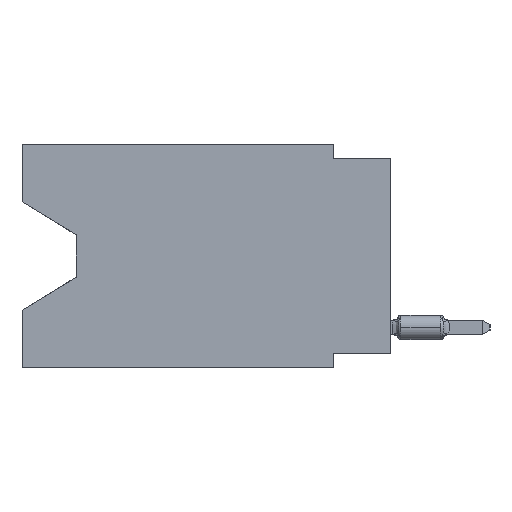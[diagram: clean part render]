
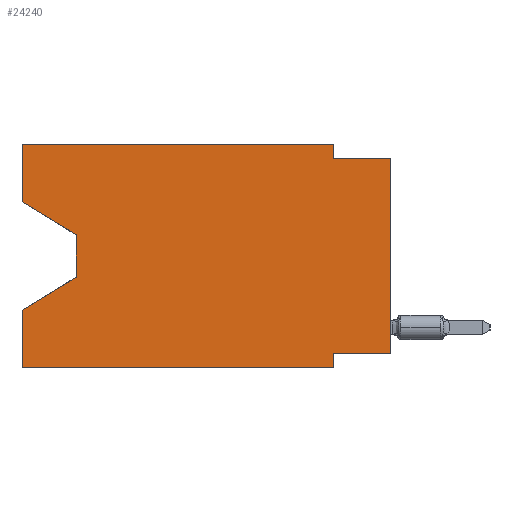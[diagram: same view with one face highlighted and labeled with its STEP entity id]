
A CAD part, left-side view. The second image highlights one B-rep face of the part: STEP entity #24240.
In plain terms, the highlighted planar face has unit normal (-1, 0, 0).
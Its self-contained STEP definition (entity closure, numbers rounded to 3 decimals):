
#132 = ORIENTED_EDGE ( 'NONE', *, *, #22557, .F. ) ;
#424 = EDGE_CURVE ( 'NONE', #26440, #10330, #9604, .T. ) ;
#500 = EDGE_CURVE ( 'NONE', #512, #4756, #3976, .T. ) ;
#512 = VERTEX_POINT ( 'NONE', #6224 ) ;
#558 = ORIENTED_EDGE ( 'NONE', *, *, #12560, .F. ) ;
#1077 = VERTEX_POINT ( 'NONE', #13866 ) ;
#1484 = EDGE_CURVE ( 'NONE', #2881, #12693, #14438, .T. ) ;
#2735 = CARTESIAN_POINT ( 'NONE',  ( 0., 13.97, -5.893 ) ) ;
#2881 = VERTEX_POINT ( 'NONE', #2735 ) ;
#3331 = ORIENTED_EDGE ( 'NONE', *, *, #6222, .F. ) ;
#3629 = VECTOR ( 'NONE', #13772, 1000. ) ;
#3734 = CARTESIAN_POINT ( 'NONE',  ( 0., 16.383, 0. ) ) ;
#3819 = ORIENTED_EDGE ( 'NONE', *, *, #23632, .F. ) ;
#3976 = LINE ( 'NONE', #12163, #6084 ) ;
#4308 = EDGE_CURVE ( 'NONE', #27775, #18327, #11653, .T. ) ;
#4413 = DIRECTION ( 'NONE',  ( 0., 0., -1. ) ) ;
#4453 = DIRECTION ( 'NONE',  ( 0., -1., 0. ) ) ;
#4756 = VERTEX_POINT ( 'NONE', #18749 ) ;
#4885 = CARTESIAN_POINT ( 'NONE',  ( 0., 16.383, 0. ) ) ;
#5933 = DIRECTION ( 'NONE',  ( 0., 0., -1. ) ) ;
#6084 = VECTOR ( 'NONE', #5933, 1000. ) ;
#6222 = EDGE_CURVE ( 'NONE', #9486, #10330, #21521, .T. ) ;
#6224 = CARTESIAN_POINT ( 'NONE',  ( 0., 2.54, -9.271 ) ) ;
#7427 = ORIENTED_EDGE ( 'NONE', *, *, #14307, .T. ) ;
#7563 = CARTESIAN_POINT ( 'NONE',  ( 0., 0., -9.271 ) ) ;
#8076 = CARTESIAN_POINT ( 'NONE',  ( 0., 2.54, 0. ) ) ;
#8082 = ORIENTED_EDGE ( 'NONE', *, *, #424, .T. ) ;
#8189 = LINE ( 'NONE', #16778, #14380 ) ;
#8214 = CARTESIAN_POINT ( 'NONE',  ( 0., 13.97, -5.893 ) ) ;
#8328 = EDGE_CURVE ( 'NONE', #18327, #9486, #8189, .T. ) ;
#9486 = VERTEX_POINT ( 'NONE', #22863 ) ;
#9604 = LINE ( 'NONE', #26800, #26778 ) ;
#9641 = VECTOR ( 'NONE', #24314, 1000. ) ;
#9661 = ORIENTED_EDGE ( 'NONE', *, *, #20714, .T. ) ;
#9950 = CARTESIAN_POINT ( 'NONE',  ( 0., 16.383, 0. ) ) ;
#10283 = CARTESIAN_POINT ( 'NONE',  ( 0., 16.383, -9.906 ) ) ;
#10330 = VERTEX_POINT ( 'NONE', #20951 ) ;
#10488 = LINE ( 'NONE', #23344, #19471 ) ;
#10808 = LINE ( 'NONE', #12367, #14360 ) ;
#11653 = LINE ( 'NONE', #4885, #9641 ) ;
#12163 = CARTESIAN_POINT ( 'NONE',  ( 0., 2.54, -9.906 ) ) ;
#12346 = VECTOR ( 'NONE', #23282, 1000. ) ;
#12367 = CARTESIAN_POINT ( 'NONE',  ( 0., 0., -9.271 ) ) ;
#12443 = VERTEX_POINT ( 'NONE', #27869 ) ;
#12560 = EDGE_CURVE ( 'NONE', #26440, #512, #10808, .T. ) ;
#12693 = VERTEX_POINT ( 'NONE', #24323 ) ;
#13282 = FACE_OUTER_BOUND ( 'NONE', #19927, .T. ) ;
#13679 = ORIENTED_EDGE ( 'NONE', *, *, #20221, .T. ) ;
#13772 = DIRECTION ( 'NONE',  ( 0., 0., 1. ) ) ;
#13803 = VECTOR ( 'NONE', #14160, 1000. ) ;
#13866 = CARTESIAN_POINT ( 'NONE',  ( 0., 16.383, -2.546 ) ) ;
#14160 = DIRECTION ( 'NONE',  ( 0., 0.855, -0.519 ) ) ;
#14307 = EDGE_CURVE ( 'NONE', #12443, #4756, #15225, .T. ) ;
#14360 = VECTOR ( 'NONE', #25306, 1000. ) ;
#14380 = VECTOR ( 'NONE', #24951, 1000. ) ;
#14438 = LINE ( 'NONE', #8214, #13803 ) ;
#15225 = LINE ( 'NONE', #10283, #21953 ) ;
#16382 = VERTEX_POINT ( 'NONE', #19220 ) ;
#16387 = DIRECTION ( 'NONE',  ( 0., 0., 1. ) ) ;
#16778 = CARTESIAN_POINT ( 'NONE',  ( 0., 2.54, 0. ) ) ;
#17148 = CARTESIAN_POINT ( 'NONE',  ( 0., 13.97, -4.013 ) ) ;
#17267 = CARTESIAN_POINT ( 'NONE',  ( 0., 0., -0.635 ) ) ;
#18327 = VERTEX_POINT ( 'NONE', #8076 ) ;
#18339 = AXIS2_PLACEMENT_3D ( 'NONE', #21888, #26368, #4413 ) ;
#18749 = CARTESIAN_POINT ( 'NONE',  ( 0., 2.54, -9.906 ) ) ;
#18832 = DIRECTION ( 'NONE',  ( 0., 0., 1. ) ) ;
#18903 = CARTESIAN_POINT ( 'NONE',  ( 0., 16.383, -2.546 ) ) ;
#19220 = CARTESIAN_POINT ( 'NONE',  ( 0., 13.97, -4.013 ) ) ;
#19272 = DIRECTION ( 'NONE',  ( 0., 0., -1. ) ) ;
#19451 = ORIENTED_EDGE ( 'NONE', *, *, #500, .F. ) ;
#19471 = VECTOR ( 'NONE', #18832, 1000. ) ;
#19927 = EDGE_LOOP ( 'NONE', ( #13679, #9661, #20577, #132, #7427, #19451, #558, #8082, #3331, #20949, #26151, #3819 ) ) ;
#20221 = EDGE_CURVE ( 'NONE', #1077, #16382, #20761, .T. ) ;
#20577 = ORIENTED_EDGE ( 'NONE', *, *, #1484, .T. ) ;
#20714 = EDGE_CURVE ( 'NONE', #16382, #2881, #24808, .T. ) ;
#20761 = LINE ( 'NONE', #18903, #12346 ) ;
#20949 = ORIENTED_EDGE ( 'NONE', *, *, #8328, .F. ) ;
#20951 = CARTESIAN_POINT ( 'NONE',  ( 0., 0., -0.635 ) ) ;
#21521 = LINE ( 'NONE', #17267, #25437 ) ;
#21888 = CARTESIAN_POINT ( 'NONE',  ( 0., 16.383, 0. ) ) ;
#21953 = VECTOR ( 'NONE', #27480, 1000. ) ;
#22557 = EDGE_CURVE ( 'NONE', #12443, #12693, #10488, .T. ) ;
#22863 = CARTESIAN_POINT ( 'NONE',  ( 0., 2.54, -0.635 ) ) ;
#23282 = DIRECTION ( 'NONE',  ( 0., -0.855, -0.519 ) ) ;
#23344 = CARTESIAN_POINT ( 'NONE',  ( 0., 16.383, 0. ) ) ;
#23632 = EDGE_CURVE ( 'NONE', #1077, #27775, #26868, .T. ) ;
#24240 = ADVANCED_FACE ( 'NONE', ( #13282 ), #25798, .F. ) ;
#24314 = DIRECTION ( 'NONE',  ( 0., -1., 0. ) ) ;
#24323 = CARTESIAN_POINT ( 'NONE',  ( 0., 16.383, -7.36 ) ) ;
#24808 = LINE ( 'NONE', #17148, #26278 ) ;
#24951 = DIRECTION ( 'NONE',  ( 0., 0., -1. ) ) ;
#25306 = DIRECTION ( 'NONE',  ( 0., 1., 0. ) ) ;
#25437 = VECTOR ( 'NONE', #4453, 1000. ) ;
#25798 = PLANE ( 'NONE',  #18339 ) ;
#26151 = ORIENTED_EDGE ( 'NONE', *, *, #4308, .F. ) ;
#26278 = VECTOR ( 'NONE', #19272, 1000. ) ;
#26368 = DIRECTION ( 'NONE',  ( 1., 0., 0. ) ) ;
#26440 = VERTEX_POINT ( 'NONE', #7563 ) ;
#26778 = VECTOR ( 'NONE', #16387, 1000. ) ;
#26800 = CARTESIAN_POINT ( 'NONE',  ( 0., 0., 0. ) ) ;
#26868 = LINE ( 'NONE', #9950, #3629 ) ;
#27480 = DIRECTION ( 'NONE',  ( 0., -1., 0. ) ) ;
#27775 = VERTEX_POINT ( 'NONE', #3734 ) ;
#27869 = CARTESIAN_POINT ( 'NONE',  ( 0., 16.383, -9.906 ) ) ;
